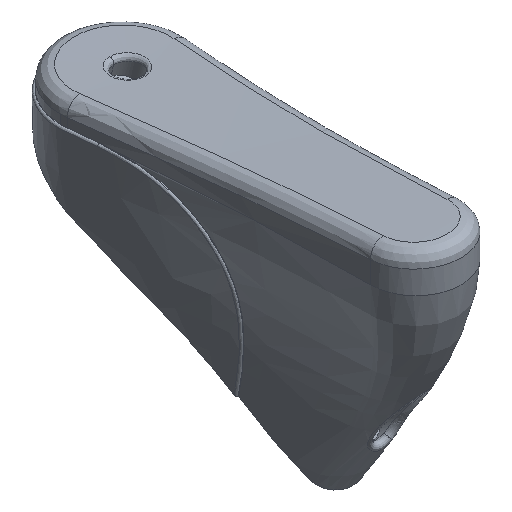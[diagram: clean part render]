
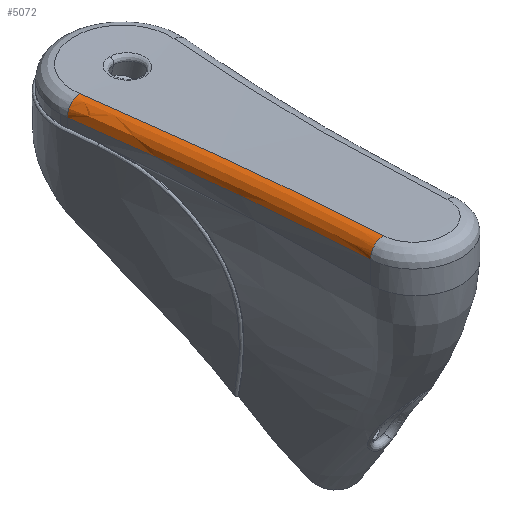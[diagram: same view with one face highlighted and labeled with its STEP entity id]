
A CAD part, isometric view. The second image highlights one B-rep face of the part: STEP entity #5072.
In plain terms, the highlighted free-form (B-spline) face has degree [3, 2] with [12, 3] control points.
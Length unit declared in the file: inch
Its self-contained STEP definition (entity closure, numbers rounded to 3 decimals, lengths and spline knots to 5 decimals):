
#79 = ORIENTED_EDGE ( 'NONE', *, *, #8667, .F. ) ;
#369 = CARTESIAN_POINT ( 'NONE',  ( -0.5757, -2.74481, 8.23349 ) ) ;
#549 = B_SPLINE_CURVE_WITH_KNOTS ( 'NONE', 3,
 ( #6428, #1838, #7809, #13774, #369, #16810, #7902, #13865, #2020, #18373, #11021, #11404 ),
 .UNSPECIFIED., .F., .F.,
 ( 4, 2, 2, 2, 2, 4 ),
 ( 0., 0.01153, 0.02305, 0.04611, 0.06916, 0.09221 ),
 .UNSPECIFIED. ) ;
#567 = DIRECTION ( 'NONE',  ( 0., 0.053, 0.999 ) ) ;
#680 = CARTESIAN_POINT ( 'NONE',  ( -0.57055, -3.18788, 8.42854 ) ) ;
#875 = CARTESIAN_POINT ( 'NONE',  ( -0.73411, -0.18185, 8.11732 ) ) ;
#902 = CARTESIAN_POINT ( 'NONE',  ( -0.59671, 0.14112, 8.28045 ) ) ;
#974 = CARTESIAN_POINT ( 'NONE',  ( -0.57, -3.5, 8.27527 ) ) ;
#1079 = CARTESIAN_POINT ( 'NONE',  ( -0.40335, -2.8847, 8.4117 ) ) ;
#1838 = CARTESIAN_POINT ( 'NONE',  ( -0.57, -3.34894, 8.26722 ) ) ;
#2020 = CARTESIAN_POINT ( 'NONE',  ( -0.65423, -1.08488, 8.14989 ) ) ;
#2058 = CARTESIAN_POINT ( 'NONE',  ( -0.57348, -2.88569, 8.41175 ) ) ;
#2133 = DIRECTION ( 'NONE',  ( -0.995, -0.105, 0. ) ) ;
#2320 = CARTESIAN_POINT ( 'NONE',  ( -0.59671, 0.13728, 8.11049 ) ) ;
#2631 =( BOUNDED_SURFACE ( )  B_SPLINE_SURFACE ( 3, 2, ( 
 ( #8220, #8416, #974 ),
 ( #8126, #15853, #3621 ),
 ( #12909, #680, #9593 ),
 ( #10970, #2058, #3711 ),
 ( #18593, #6744, #16941 ),
 ( #12711, #9500, #9685 ),
 ( #18690, #3809, #14088 ),
 ( #9784, #3906, #15560 ),
 ( #18502, #14279, #8029 ),
 ( #15754, #15653, #5085 ),
 ( #5176, #8316, #875 ),
 ( #13994, #6845, #11060 ) ),
 .UNSPECIFIED., .F., .F., .T. ) 
 B_SPLINE_SURFACE_WITH_KNOTS ( ( 4, 2, 2, 2, 2, 4 ),
 ( 3, 3 ),
 ( 0., 0.01158, 0.02317, 0.04633, 0.0695, 0.09267 ),
 ( 0., 1. ),
 .UNSPECIFIED. ) 
 GEOMETRIC_REPRESENTATION_ITEM ( )  RATIONAL_B_SPLINE_SURFACE ( (
 ( 1., 0.707, 1.),
 ( 1., 0.707, 1.),
 ( 1., 0.707, 1.),
 ( 1., 0.707, 1.),
 ( 1., 0.707, 1.),
 ( 1., 0.706, 1.),
 ( 1., 0.706, 1.),
 ( 1., 0.706, 1.),
 ( 1., 0.706, 1.),
 ( 1., 0.706, 1.),
 ( 1., 0.706, 1.),
 ( 1., 0.706, 1.) ) ) 
 REPRESENTATION_ITEM ( '' )  SURFACE ( )  );
#3621 = CARTESIAN_POINT ( 'NONE',  ( -0.57, -3.34855, 8.2672 ) ) ;
#3711 = CARTESIAN_POINT ( 'NONE',  ( -0.57335, -2.89515, 8.24189 ) ) ;
#3809 = CARTESIAN_POINT ( 'NONE',  ( -0.59883, -1.98143, 8.36282 ) ) ;
#3906 = CARTESIAN_POINT ( 'NONE',  ( -0.63289, -1.37959, 8.33367 ) ) ;
#4110 = CARTESIAN_POINT ( 'NONE',  ( -0.40571, -2.73315, 8.40327 ) ) ;
#4230 = ORIENTED_EDGE ( 'NONE', *, *, #5679, .F. ) ;
#4310 = AXIS2_PLACEMENT_3D ( 'NONE', #8008, #12594, #567 ) ;
#5072 = ADVANCED_FACE ( 'NONE', ( #12525 ), #2631, .T. ) ;
#5085 = CARTESIAN_POINT ( 'NONE',  ( -0.70503, -0.48318, 8.12694 ) ) ;
#5176 = CARTESIAN_POINT ( 'NONE',  ( -0.56494, -0.16015, 8.28725 ) ) ;
#5281 = CARTESIAN_POINT ( 'NONE',  ( -0.46262, -1.37002, 8.33323 ) ) ;
#5501 = CARTESIAN_POINT ( 'NONE',  ( -0.57, -3.5, 8.27527 ) ) ;
#5508 = B_SPLINE_CURVE_WITH_KNOTS ( 'NONE', 3,
 ( #14586, #15960, #18695, #8522, #5281, #17525, #14386, #4110, #1079, #11255, #14487, #17227 ),
 .UNSPECIFIED., .F., .F.,
 ( 4, 2, 2, 2, 2, 4 ),
 ( 0., 0.02313, 0.04627, 0.0694, 0.08097, 0.09254 ),
 .UNSPECIFIED. ) ;
#5679 = EDGE_CURVE ( 'NONE', #7172, #13035, #12135, .T. ) ;
#6033 = EDGE_CURVE ( 'NONE', #13233, #11632, #11490, .T. ) ;
#6428 = CARTESIAN_POINT ( 'NONE',  ( -0.57, -3.5, 8.27527 ) ) ;
#6744 = CARTESIAN_POINT ( 'NONE',  ( -0.57588, -2.73482, 8.40337 ) ) ;
#6845 = CARTESIAN_POINT ( 'NONE',  ( -0.76618, 0.12332, 8.28085 ) ) ;
#7172 = VERTEX_POINT ( 'NONE', #11851 ) ;
#7809 = CARTESIAN_POINT ( 'NONE',  ( -0.5705, -3.19788, 8.25878 ) ) ;
#7902 = CARTESIAN_POINT ( 'NONE',  ( -0.59844, -1.98981, 8.19262 ) ) ;
#8008 = CARTESIAN_POINT ( 'NONE',  ( -0.4, -3.5, 8.27527 ) ) ;
#8029 = CARTESIAN_POINT ( 'NONE',  ( -0.65414, -1.08596, 8.14993 ) ) ;
#8126 = CARTESIAN_POINT ( 'NONE',  ( -0.4, -3.33885, 8.43694 ) ) ;
#8220 = CARTESIAN_POINT ( 'NONE',  ( -0.4, -3.49098, 8.44503 ) ) ;
#8292 = DIRECTION ( 'NONE',  ( -0.105, 0.994, -0.022 ) ) ;
#8316 = CARTESIAN_POINT ( 'NONE',  ( -0.73459, -0.17706, 8.28774 ) ) ;
#8416 = CARTESIAN_POINT ( 'NONE',  ( -0.57, -3.49098, 8.44503 ) ) ;
#8522 = CARTESIAN_POINT ( 'NONE',  ( -0.48451, -1.06744, 8.31985 ) ) ;
#8667 = EDGE_CURVE ( 'NONE', #13233, #7172, #549, .T. ) ;
#9500 = CARTESIAN_POINT ( 'NONE',  ( -0.58669, -2.2825, 8.37867 ) ) ;
#9593 = CARTESIAN_POINT ( 'NONE',  ( -0.5705, -3.19732, 8.25875 ) ) ;
#9685 = CARTESIAN_POINT ( 'NONE',  ( -0.58638, -2.29164, 8.2086 ) ) ;
#9784 = CARTESIAN_POINT ( 'NONE',  ( -0.46274, -1.36829, 8.33315 ) ) ;
#10970 = CARTESIAN_POINT ( 'NONE',  ( -0.40336, -2.88341, 8.41163 ) ) ;
#11021 = CARTESIAN_POINT ( 'NONE',  ( -0.73417, -0.18129, 8.1173 ) ) ;
#11060 = CARTESIAN_POINT ( 'NONE',  ( -0.76578, 0.11951, 8.11049 ) ) ;
#11180 = AXIS2_PLACEMENT_3D ( 'NONE', #2320, #8292, #2133 ) ;
#11255 = CARTESIAN_POINT ( 'NONE',  ( -0.4005, -3.18781, 8.42853 ) ) ;
#11404 = CARTESIAN_POINT ( 'NONE',  ( -0.76578, 0.11951, 8.11049 ) ) ;
#11490 = CIRCLE ( 'NONE', #4310, 0.17 ) ;
#11632 = VERTEX_POINT ( 'NONE', #16710 ) ;
#11851 = CARTESIAN_POINT ( 'NONE',  ( -0.76578, 0.11951, 8.11049 ) ) ;
#12135 = CIRCLE ( 'NONE', #11180, 0.17 ) ;
#12525 = FACE_OUTER_BOUND ( 'NONE', #18193, .T. ) ;
#12594 = DIRECTION ( 'NONE',  ( 0., 0.999, -0.053 ) ) ;
#12711 = CARTESIAN_POINT ( 'NONE',  ( -0.41647, -2.2768, 8.37836 ) ) ;
#12909 = CARTESIAN_POINT ( 'NONE',  ( -0.4005, -3.18698, 8.42849 ) ) ;
#13035 = VERTEX_POINT ( 'NONE', #902 ) ;
#13233 = VERTEX_POINT ( 'NONE', #5501 ) ;
#13774 = CARTESIAN_POINT ( 'NONE',  ( -0.57334, -2.89582, 8.24193 ) ) ;
#13865 = CARTESIAN_POINT ( 'NONE',  ( -0.63243, -1.38642, 8.16328 ) ) ;
#13994 = CARTESIAN_POINT ( 'NONE',  ( -0.59671, 0.14112, 8.28045 ) ) ;
#14088 = CARTESIAN_POINT ( 'NONE',  ( -0.59842, -1.99016, 8.19264 ) ) ;
#14172 = EDGE_CURVE ( 'NONE', #13035, #11632, #5508, .T. ) ;
#14279 = CARTESIAN_POINT ( 'NONE',  ( -0.65469, -1.07882, 8.32033 ) ) ;
#14386 = CARTESIAN_POINT ( 'NONE',  ( -0.41641, -2.27856, 8.37845 ) ) ;
#14487 = CARTESIAN_POINT ( 'NONE',  ( -0.4, -3.33938, 8.43697 ) ) ;
#14586 = CARTESIAN_POINT ( 'NONE',  ( -0.59671, 0.14112, 8.28045 ) ) ;
#14905 = ORIENTED_EDGE ( 'NONE', *, *, #6033, .T. ) ;
#15560 = CARTESIAN_POINT ( 'NONE',  ( -0.63237, -1.38738, 8.16332 ) ) ;
#15653 = CARTESIAN_POINT ( 'NONE',  ( -0.70557, -0.47748, 8.29738 ) ) ;
#15754 = CARTESIAN_POINT ( 'NONE',  ( -0.53575, -0.46178, 8.29684 ) ) ;
#15853 = CARTESIAN_POINT ( 'NONE',  ( -0.57002, -3.33921, 8.43696 ) ) ;
#15960 = CARTESIAN_POINT ( 'NONE',  ( -0.56487, -0.16077, 8.28726 ) ) ;
#16710 = CARTESIAN_POINT ( 'NONE',  ( -0.4, -3.49098, 8.44503 ) ) ;
#16810 = CARTESIAN_POINT ( 'NONE',  ( -0.58637, -2.29179, 8.20861 ) ) ;
#16941 = CARTESIAN_POINT ( 'NONE',  ( -0.57571, -2.74422, 8.23345 ) ) ;
#17227 = CARTESIAN_POINT ( 'NONE',  ( -0.4, -3.49098, 8.44503 ) ) ;
#17525 = CARTESIAN_POINT ( 'NONE',  ( -0.42851, -1.97552, 8.36251 ) ) ;
#18037 = ORIENTED_EDGE ( 'NONE', *, *, #14172, .F. ) ;
#18193 = EDGE_LOOP ( 'NONE', ( #14905, #18037, #4230, #79 ) ) ;
#18373 = CARTESIAN_POINT ( 'NONE',  ( -0.70511, -0.48234, 8.12691 ) ) ;
#18502 = CARTESIAN_POINT ( 'NONE',  ( -0.48463, -1.06585, 8.31978 ) ) ;
#18593 = CARTESIAN_POINT ( 'NONE',  ( -0.40574, -2.73172, 8.40319 ) ) ;
#18690 = CARTESIAN_POINT ( 'NONE',  ( -0.42859, -1.97371, 8.36242 ) ) ;
#18695 = CARTESIAN_POINT ( 'NONE',  ( -0.53565, -0.46281, 8.29688 ) ) ;
